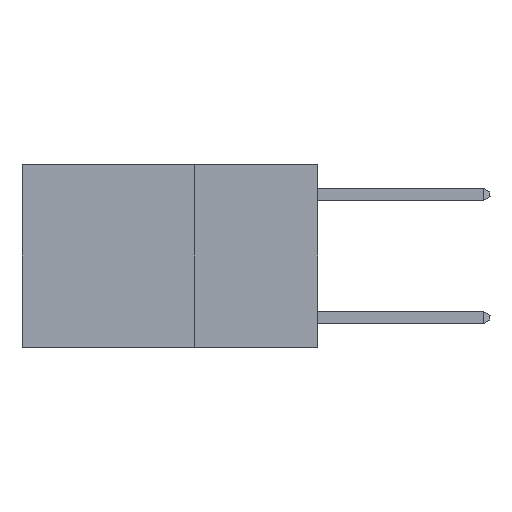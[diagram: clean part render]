
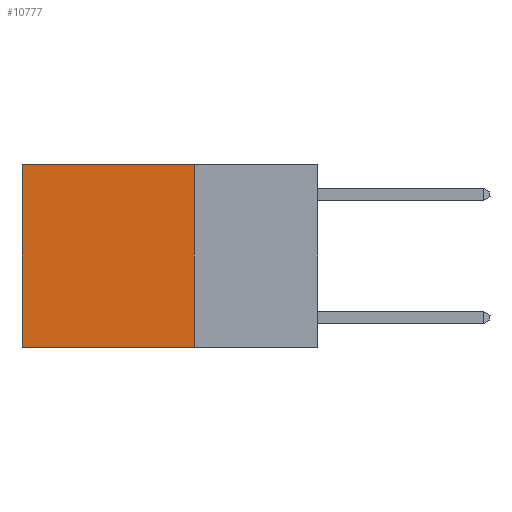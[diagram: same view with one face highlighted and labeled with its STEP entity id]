
A CAD part, left-side view. The second image highlights one B-rep face of the part: STEP entity #10777.
In plain terms, the highlighted planar face has unit normal (-1, 0, 0).
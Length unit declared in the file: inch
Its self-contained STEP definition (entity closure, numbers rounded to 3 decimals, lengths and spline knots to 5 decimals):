
#117 = ORIENTED_EDGE ( 'NONE', *, *, #7752, .F. ) ;
#786 = VERTEX_POINT ( 'NONE', #8343 ) ;
#1500 = ORIENTED_EDGE ( 'NONE', *, *, #5551, .T. ) ;
#1539 = DIRECTION ( 'NONE',  ( 0., 0., -1. ) ) ;
#1546 = VECTOR ( 'NONE', #1539, 39.37008 ) ;
#2133 = DIRECTION ( 'NONE',  ( 0., 0., -1. ) ) ;
#2237 = CARTESIAN_POINT ( 'NONE',  ( 0.2625, 0.25, 0. ) ) ;
#2268 = CARTESIAN_POINT ( 'NONE',  ( 0.2625, 0.25, 0. ) ) ;
#2389 = DIRECTION ( 'NONE',  ( 0., 1., 0. ) ) ;
#2618 = AXIS2_PLACEMENT_3D ( 'NONE', #2268, #9189, #9943 ) ;
#2699 = VERTEX_POINT ( 'NONE', #12379 ) ;
#3279 = LINE ( 'NONE', #10755, #11411 ) ;
#3384 = LINE ( 'NONE', #6473, #1546 ) ;
#4073 = VECTOR ( 'NONE', #4810, 39.37008 ) ;
#4133 = CARTESIAN_POINT ( 'NONE',  ( 0.2625, 0.25, -0.37 ) ) ;
#4681 = CARTESIAN_POINT ( 'NONE',  ( 0.2625, 0.25, 0. ) ) ;
#4810 = DIRECTION ( 'NONE',  ( 0., 1., 0. ) ) ;
#5300 = VERTEX_POINT ( 'NONE', #2237 ) ;
#5484 = LINE ( 'NONE', #9261, #7481 ) ;
#5551 = EDGE_CURVE ( 'NONE', #5300, #2699, #5829, .T. ) ;
#5829 = LINE ( 'NONE', #4681, #4073 ) ;
#6305 = PLANE ( 'NONE',  #2618 ) ;
#6473 = CARTESIAN_POINT ( 'NONE',  ( 0.2625, 0.25, 0. ) ) ;
#6795 = EDGE_CURVE ( 'NONE', #5300, #11912, #3384, .T. ) ;
#7268 = ORIENTED_EDGE ( 'NONE', *, *, #6795, .F. ) ;
#7449 = EDGE_LOOP ( 'NONE', ( #10222, #117, #7268, #1500 ) ) ;
#7481 = VECTOR ( 'NONE', #2389, 39.37008 ) ;
#7752 = EDGE_CURVE ( 'NONE', #11912, #786, #5484, .T. ) ;
#8343 = CARTESIAN_POINT ( 'NONE',  ( 0.2625, 0.6, -0.37 ) ) ;
#8451 = FACE_OUTER_BOUND ( 'NONE', #7449, .T. ) ;
#9007 = EDGE_CURVE ( 'NONE', #2699, #786, #3279, .T. ) ;
#9189 = DIRECTION ( 'NONE',  ( 1., 0., 0. ) ) ;
#9261 = CARTESIAN_POINT ( 'NONE',  ( 0.2625, 0.25, -0.37 ) ) ;
#9943 = DIRECTION ( 'NONE',  ( 0., 0., -1. ) ) ;
#10222 = ORIENTED_EDGE ( 'NONE', *, *, #9007, .T. ) ;
#10755 = CARTESIAN_POINT ( 'NONE',  ( 0.2625, 0.6, 0. ) ) ;
#10777 = ADVANCED_FACE ( 'NONE', ( #8451 ), #6305, .F. ) ;
#11411 = VECTOR ( 'NONE', #2133, 39.37008 ) ;
#11912 = VERTEX_POINT ( 'NONE', #4133 ) ;
#12379 = CARTESIAN_POINT ( 'NONE',  ( 0.2625, 0.6, 0. ) ) ;
